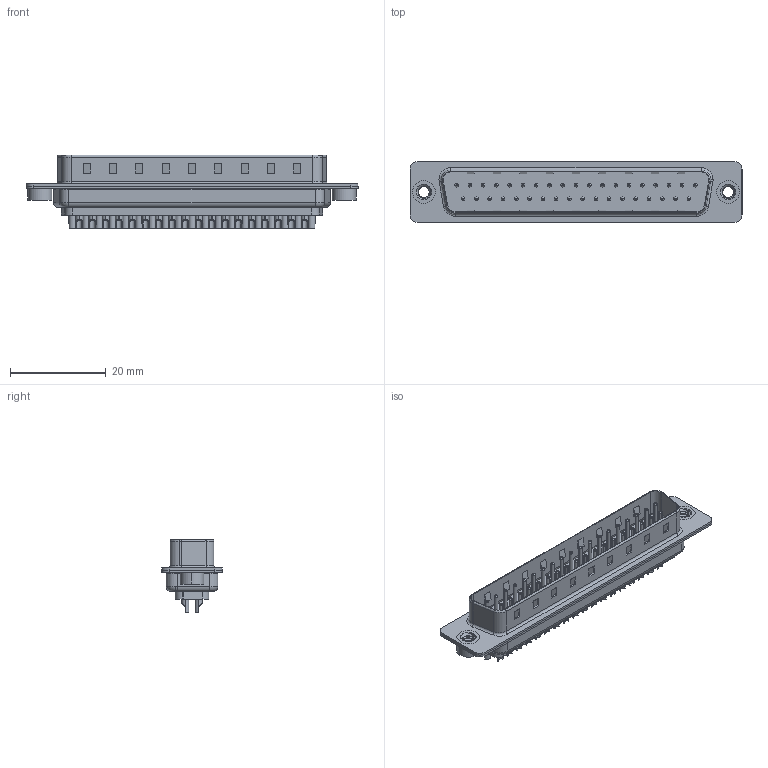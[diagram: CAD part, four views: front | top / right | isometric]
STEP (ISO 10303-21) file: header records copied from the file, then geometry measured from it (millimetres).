
FILE_DESCRIPTION (( 'STEP AP203' ), '1' );
FILE_NAME ('627-037-622-242.STEP', '2020-07-15T08:42:29', ( '' ), ( '' ), 'SwSTEP 2.0', 'SolidWorks 2020', '' );
FILE_SCHEMA (( 'CONFIG_CONTROL_DESIGN' ));
Length unit declared in the file: millimetre
Products named in the file (7): 627-037-622-242; 627 Contact Row 1_22L; 627 4-40 Threaded Rivet; 627 Shell Front_37 Contacts; 627 Shell Rear_37 Contacts; 627 Contact Row 2_22L; 627 Housing_37 LP
Assembly tree (42 placements, depth 2):
  627-037-622-242
    627 Housing_37 LP
    627 Shell Front_37 Contacts
    627 Shell Rear_37 Contacts
    627 Contact Row 1_22L  x19
    627 Contact Row 2_22L  x18
    627 4-40 Threaded Rivet  x2
Bounding box: 69.3 x 12.6 x 15.35 mm (x, y, z)
Volume: 3709.4 mm3; surface area: 10746.6 mm2
Topology: 42 solids, 42 shells, 2776 faces, 7115 edges, 4508 vertices
Faces by surface type: cylinder 1212, torus 827, plane 721, cone 10, bspline 6
Entity records: 26933 total; most frequent: CARTESIAN_POINT 5604, DIRECTION 4422, ORIENTED_EDGE 3858, EDGE_CURVE 1929, AXIS2_PLACEMENT_3D 1735, VERTEX_POINT 1239, EDGE_LOOP 992, VECTOR 952
